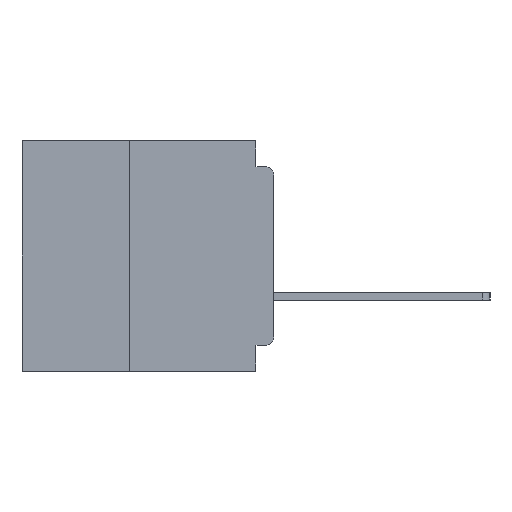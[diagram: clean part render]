
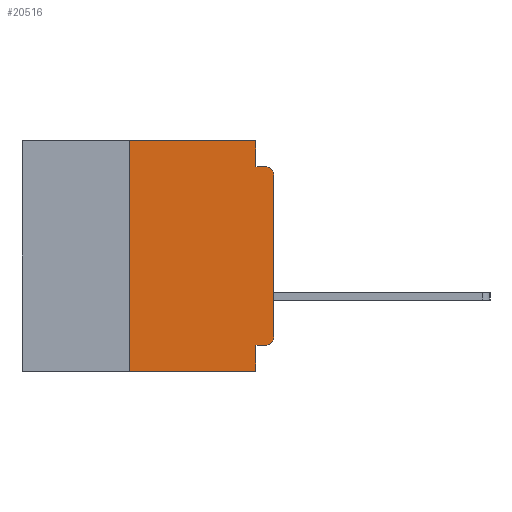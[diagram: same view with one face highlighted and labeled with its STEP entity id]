
A CAD part, left-side view. The second image highlights one B-rep face of the part: STEP entity #20516.
In plain terms, the highlighted planar face has unit normal (-1, 0, 0).
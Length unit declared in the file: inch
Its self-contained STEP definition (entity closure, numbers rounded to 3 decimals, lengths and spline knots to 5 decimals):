
#119 = EDGE_CURVE ( 'NONE', #295, #20531, #26899, .T. ) ;
#295 = VERTEX_POINT ( 'NONE', #26319 ) ;
#2038 = LINE ( 'NONE', #9011, #18892 ) ;
#4444 = EDGE_CURVE ( 'NONE', #37694, #14412, #29134, .T. ) ;
#5147 = DIRECTION ( 'NONE',  ( -1., 0., 0. ) ) ;
#5569 = CARTESIAN_POINT ( 'NONE',  ( 0., 0.437, 0. ) ) ;
#6308 = VECTOR ( 'NONE', #33315, 39.37008 ) ;
#6625 = ORIENTED_EDGE ( 'NONE', *, *, #22183, .T. ) ;
#7219 = ORIENTED_EDGE ( 'NONE', *, *, #29080, .T. ) ;
#7238 = CIRCLE ( 'NONE', #15666, 0.015 ) ;
#7439 = LINE ( 'NONE', #11685, #17456 ) ;
#7907 = EDGE_LOOP ( 'NONE', ( #6625, #7219, #8286, #10969, #12010, #12683, #13111, #16763, #17956, #22186 ) ) ;
#8051 = VECTOR ( 'NONE', #20134, 39.37008 ) ;
#8078 = VERTEX_POINT ( 'NONE', #19828 ) ;
#8103 = EDGE_CURVE ( 'NONE', #37694, #8078, #15298, .T. ) ;
#8286 = ORIENTED_EDGE ( 'NONE', *, *, #23013, .F. ) ;
#8365 = VECTOR ( 'NONE', #30893, 39.37008 ) ;
#8587 = LINE ( 'NONE', #33784, #16516 ) ;
#9011 = CARTESIAN_POINT ( 'NONE',  ( 0., 0.25, -0.4 ) ) ;
#10408 = VECTOR ( 'NONE', #32920, 39.37008 ) ;
#10969 = ORIENTED_EDGE ( 'NONE', *, *, #119, .F. ) ;
#11593 = LINE ( 'NONE', #5569, #36015 ) ;
#11685 = CARTESIAN_POINT ( 'NONE',  ( 0., 0.031, -0.4 ) ) ;
#12010 = ORIENTED_EDGE ( 'NONE', *, *, #13052, .F. ) ;
#12127 = DIRECTION ( 'NONE',  ( 1., 0., 0. ) ) ;
#12277 = EDGE_CURVE ( 'NONE', #8078, #33772, #7439, .T. ) ;
#12683 = ORIENTED_EDGE ( 'NONE', *, *, #32335, .F. ) ;
#13052 = EDGE_CURVE ( 'NONE', #29733, #295, #11593, .T. ) ;
#13111 = ORIENTED_EDGE ( 'NONE', *, *, #25676, .T. ) ;
#13877 = DIRECTION ( 'NONE',  ( 0., -1., 0. ) ) ;
#14412 = VERTEX_POINT ( 'NONE', #40316 ) ;
#15108 = DIRECTION ( 'NONE',  ( 0., 0., -1. ) ) ;
#15298 = LINE ( 'NONE', #29973, #6308 ) ;
#15612 = DIRECTION ( 'NONE',  ( 0., -1., 0. ) ) ;
#15666 = AXIS2_PLACEMENT_3D ( 'NONE', #25230, #5147, #28529 ) ;
#16516 = VECTOR ( 'NONE', #13877, 39.37008 ) ;
#16763 = ORIENTED_EDGE ( 'NONE', *, *, #12277, .F. ) ;
#17358 = LINE ( 'NONE', #27562, #8365 ) ;
#17456 = VECTOR ( 'NONE', #15108, 39.37008 ) ;
#17956 = ORIENTED_EDGE ( 'NONE', *, *, #8103, .F. ) ;
#18730 = PLANE ( 'NONE',  #25705 ) ;
#18892 = VECTOR ( 'NONE', #38984, 39.37008 ) ;
#19357 = LINE ( 'NONE', #26258, #10408 ) ;
#19828 = CARTESIAN_POINT ( 'NONE',  ( 0., 0.031, -0.355 ) ) ;
#20134 = DIRECTION ( 'NONE',  ( 0., 0., -1. ) ) ;
#20237 = CARTESIAN_POINT ( 'NONE',  ( 0., 0.031, -0.4 ) ) ;
#20516 = ADVANCED_FACE ( 'NONE', ( #35137 ), #18730, .F. ) ;
#20531 = VERTEX_POINT ( 'NONE', #25537 ) ;
#21976 = CARTESIAN_POINT ( 'NONE',  ( 0., 0.25, 0. ) ) ;
#22058 = CARTESIAN_POINT ( 'NONE',  ( 0., 0.437, 0. ) ) ;
#22183 = EDGE_CURVE ( 'NONE', #14412, #24187, #17358, .T. ) ;
#22186 = ORIENTED_EDGE ( 'NONE', *, *, #4444, .T. ) ;
#23013 = EDGE_CURVE ( 'NONE', #20531, #38458, #19357, .T. ) ;
#24187 = VERTEX_POINT ( 'NONE', #29174 ) ;
#24790 = CARTESIAN_POINT ( 'NONE',  ( 0., 0.015, -0.355 ) ) ;
#25230 = CARTESIAN_POINT ( 'NONE',  ( 0., 0.015, -0.06 ) ) ;
#25537 = CARTESIAN_POINT ( 'NONE',  ( 0., 0.031, -0.045 ) ) ;
#25676 = EDGE_CURVE ( 'NONE', #33839, #33772, #8587, .T. ) ;
#25705 = AXIS2_PLACEMENT_3D ( 'NONE', #22058, #12127, #35359 ) ;
#26258 = CARTESIAN_POINT ( 'NONE',  ( 0., 0., -0.045 ) ) ;
#26319 = CARTESIAN_POINT ( 'NONE',  ( 0., 0.031, 0. ) ) ;
#26899 = LINE ( 'NONE', #28501, #8051 ) ;
#27562 = CARTESIAN_POINT ( 'NONE',  ( 0., 0., 0. ) ) ;
#28501 = CARTESIAN_POINT ( 'NONE',  ( 0., 0.031, 0. ) ) ;
#28529 = DIRECTION ( 'NONE',  ( 0., 0., -1. ) ) ;
#29080 = EDGE_CURVE ( 'NONE', #24187, #38458, #7238, .T. ) ;
#29134 = CIRCLE ( 'NONE', #31866, 0.015 ) ;
#29174 = CARTESIAN_POINT ( 'NONE',  ( 0., 0., -0.06 ) ) ;
#29733 = VERTEX_POINT ( 'NONE', #21976 ) ;
#29973 = CARTESIAN_POINT ( 'NONE',  ( 0., 0., -0.355 ) ) ;
#30893 = DIRECTION ( 'NONE',  ( 0., 0., 1. ) ) ;
#31154 = DIRECTION ( 'NONE',  ( 0., 0., -1. ) ) ;
#31182 = DIRECTION ( 'NONE',  ( -1., 0., 0. ) ) ;
#31236 = CARTESIAN_POINT ( 'NONE',  ( 0., 0.015, -0.34 ) ) ;
#31866 = AXIS2_PLACEMENT_3D ( 'NONE', #31236, #31182, #31154 ) ;
#32066 = CARTESIAN_POINT ( 'NONE',  ( 0., 0.015, -0.045 ) ) ;
#32173 = CARTESIAN_POINT ( 'NONE',  ( 0., 0.25, -0.4 ) ) ;
#32335 = EDGE_CURVE ( 'NONE', #33839, #29733, #2038, .T. ) ;
#32920 = DIRECTION ( 'NONE',  ( 0., -1., 0. ) ) ;
#33315 = DIRECTION ( 'NONE',  ( 0., 1., 0. ) ) ;
#33772 = VERTEX_POINT ( 'NONE', #20237 ) ;
#33784 = CARTESIAN_POINT ( 'NONE',  ( 0., 0.437, -0.4 ) ) ;
#33839 = VERTEX_POINT ( 'NONE', #32173 ) ;
#35137 = FACE_OUTER_BOUND ( 'NONE', #7907, .T. ) ;
#35359 = DIRECTION ( 'NONE',  ( 0., 0., -1. ) ) ;
#36015 = VECTOR ( 'NONE', #15612, 39.37008 ) ;
#37694 = VERTEX_POINT ( 'NONE', #24790 ) ;
#38458 = VERTEX_POINT ( 'NONE', #32066 ) ;
#38984 = DIRECTION ( 'NONE',  ( 0., 0., 1. ) ) ;
#40316 = CARTESIAN_POINT ( 'NONE',  ( 0., 0., -0.34 ) ) ;
